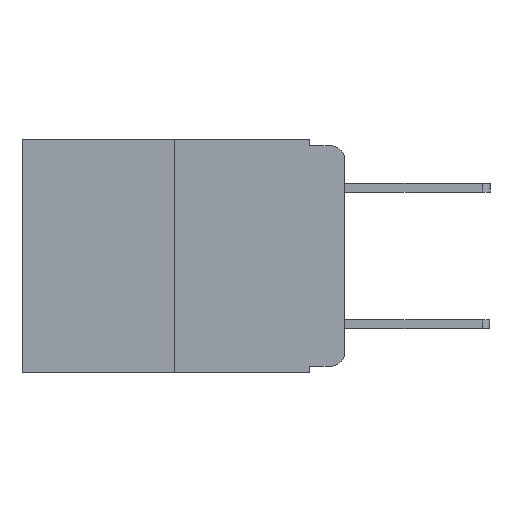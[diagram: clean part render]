
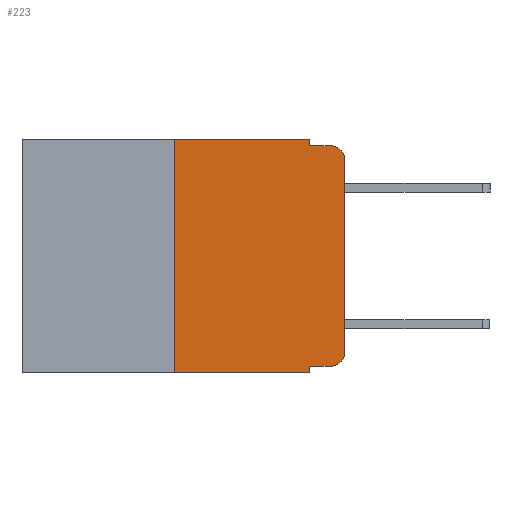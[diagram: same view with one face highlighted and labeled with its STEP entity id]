
A CAD part, left-side view. The second image highlights one B-rep face of the part: STEP entity #223.
In plain terms, the highlighted planar face has unit normal (-1, 0, 0).
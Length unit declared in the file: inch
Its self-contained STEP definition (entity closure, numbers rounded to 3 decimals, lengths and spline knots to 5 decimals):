
#196 = CARTESIAN_POINT ( 'NONE',  ( 0., 0.473, -0.343 ) ) ;
#216 = VERTEX_POINT ( 'NONE', #3638 ) ;
#223 = ADVANCED_FACE ( 'NONE', ( #1597 ), #9440, .F. ) ;
#251 = VERTEX_POINT ( 'NONE', #6476 ) ;
#408 = CARTESIAN_POINT ( 'NONE',  ( 0., 0.051, -0.01 ) ) ;
#806 = EDGE_CURVE ( 'NONE', #216, #2228, #10338, .T. ) ;
#811 = ORIENTED_EDGE ( 'NONE', *, *, #6741, .F. ) ;
#897 = DIRECTION ( 'NONE',  ( -1., 0., 0. ) ) ;
#949 = AXIS2_PLACEMENT_3D ( 'NONE', #9639, #4742, #10482 ) ;
#1180 = EDGE_CURVE ( 'NONE', #251, #8463, #7514, .T. ) ;
#1597 = FACE_OUTER_BOUND ( 'NONE', #4445, .T. ) ;
#1632 = LINE ( 'NONE', #1672, #9632 ) ;
#1672 = CARTESIAN_POINT ( 'NONE',  ( 0., 0.051, -0.01 ) ) ;
#1817 = CARTESIAN_POINT ( 'NONE',  ( 0., 0.02, -0.313 ) ) ;
#1845 = AXIS2_PLACEMENT_3D ( 'NONE', #7605, #2229, #7422 ) ;
#1893 = CARTESIAN_POINT ( 'NONE',  ( 0., 0.051, 0. ) ) ;
#1928 = CARTESIAN_POINT ( 'NONE',  ( 0., 0.051, -0.333 ) ) ;
#2087 = ORIENTED_EDGE ( 'NONE', *, *, #3782, .T. ) ;
#2106 = VECTOR ( 'NONE', #9404, 39.37008 ) ;
#2228 = VERTEX_POINT ( 'NONE', #7787 ) ;
#2229 = DIRECTION ( 'NONE',  ( 1., 0., 0. ) ) ;
#2386 = ORIENTED_EDGE ( 'NONE', *, *, #806, .F. ) ;
#2463 = DIRECTION ( 'NONE',  ( 0., -1., 0. ) ) ;
#2829 = DIRECTION ( 'NONE',  ( 0., 0., -1. ) ) ;
#2911 = VECTOR ( 'NONE', #5939, 39.37008 ) ;
#3011 = CARTESIAN_POINT ( 'NONE',  ( 0., 0., -0.313 ) ) ;
#3073 = VECTOR ( 'NONE', #9023, 39.37008 ) ;
#3480 = DIRECTION ( 'NONE',  ( 0., -1., 0. ) ) ;
#3638 = CARTESIAN_POINT ( 'NONE',  ( 0., 0.25, 0. ) ) ;
#3747 = VERTEX_POINT ( 'NONE', #6736 ) ;
#3782 = EDGE_CURVE ( 'NONE', #6854, #10087, #6702, .T. ) ;
#3838 = CIRCLE ( 'NONE', #949, 0.02 ) ;
#3851 = VECTOR ( 'NONE', #3480, 39.37008 ) ;
#4028 = CARTESIAN_POINT ( 'NONE',  ( 0., 0.051, 0. ) ) ;
#4170 = EDGE_CURVE ( 'NONE', #5185, #3747, #1632, .T. ) ;
#4412 = AXIS2_PLACEMENT_3D ( 'NONE', #1817, #897, #10170 ) ;
#4445 = EDGE_LOOP ( 'NONE', ( #8730, #10282, #5439, #811, #2386, #7401, #9883, #6822, #10832, #2087 ) ) ;
#4742 = DIRECTION ( 'NONE',  ( -1., 0., 0. ) ) ;
#4751 = EDGE_CURVE ( 'NONE', #4864, #216, #5285, .T. ) ;
#4757 = CARTESIAN_POINT ( 'NONE',  ( 0., 0.02, -0.333 ) ) ;
#4864 = VERTEX_POINT ( 'NONE', #6947 ) ;
#5097 = VECTOR ( 'NONE', #2829, 39.37008 ) ;
#5185 = VERTEX_POINT ( 'NONE', #408 ) ;
#5285 = LINE ( 'NONE', #7669, #2911 ) ;
#5436 = LINE ( 'NONE', #8190, #3073 ) ;
#5439 = ORIENTED_EDGE ( 'NONE', *, *, #4170, .F. ) ;
#5939 = DIRECTION ( 'NONE',  ( 0., 0., 1. ) ) ;
#6011 = VECTOR ( 'NONE', #2463, 39.37008 ) ;
#6476 = CARTESIAN_POINT ( 'NONE',  ( 0., 0.051, -0.333 ) ) ;
#6702 = CIRCLE ( 'NONE', #4412, 0.02 ) ;
#6736 = CARTESIAN_POINT ( 'NONE',  ( 0., 0.02, -0.01 ) ) ;
#6741 = EDGE_CURVE ( 'NONE', #2228, #5185, #10964, .T. ) ;
#6822 = ORIENTED_EDGE ( 'NONE', *, *, #1180, .F. ) ;
#6854 = VERTEX_POINT ( 'NONE', #4757 ) ;
#6899 = VECTOR ( 'NONE', #8946, 39.37008 ) ;
#6947 = CARTESIAN_POINT ( 'NONE',  ( 0., 0.25, -0.343 ) ) ;
#7375 = EDGE_CURVE ( 'NONE', #251, #6854, #9168, .T. ) ;
#7401 = ORIENTED_EDGE ( 'NONE', *, *, #4751, .F. ) ;
#7422 = DIRECTION ( 'NONE',  ( 0., 0., -1. ) ) ;
#7474 = EDGE_CURVE ( 'NONE', #4864, #8463, #8238, .T. ) ;
#7514 = LINE ( 'NONE', #4028, #5097 ) ;
#7605 = CARTESIAN_POINT ( 'NONE',  ( 0., 0.473, 0. ) ) ;
#7669 = CARTESIAN_POINT ( 'NONE',  ( 0., 0.25, 0. ) ) ;
#7787 = CARTESIAN_POINT ( 'NONE',  ( 0., 0.051, 0. ) ) ;
#7907 = EDGE_CURVE ( 'NONE', #9501, #3747, #3838, .T. ) ;
#7925 = CARTESIAN_POINT ( 'NONE',  ( 0., 0., -0.03 ) ) ;
#8190 = CARTESIAN_POINT ( 'NONE',  ( 0., 0., 0. ) ) ;
#8238 = LINE ( 'NONE', #196, #3851 ) ;
#8317 = CARTESIAN_POINT ( 'NONE',  ( 0., 0.051, -0.343 ) ) ;
#8463 = VERTEX_POINT ( 'NONE', #8317 ) ;
#8730 = ORIENTED_EDGE ( 'NONE', *, *, #9913, .T. ) ;
#8946 = DIRECTION ( 'NONE',  ( 0., 0., -1. ) ) ;
#9023 = DIRECTION ( 'NONE',  ( 0., 0., 1. ) ) ;
#9168 = LINE ( 'NONE', #1928, #2106 ) ;
#9404 = DIRECTION ( 'NONE',  ( 0., -1., 0. ) ) ;
#9440 = PLANE ( 'NONE',  #1845 ) ;
#9501 = VERTEX_POINT ( 'NONE', #7925 ) ;
#9632 = VECTOR ( 'NONE', #10300, 39.37008 ) ;
#9639 = CARTESIAN_POINT ( 'NONE',  ( 0., 0.02, -0.03 ) ) ;
#9883 = ORIENTED_EDGE ( 'NONE', *, *, #7474, .T. ) ;
#9913 = EDGE_CURVE ( 'NONE', #10087, #9501, #5436, .T. ) ;
#10087 = VERTEX_POINT ( 'NONE', #3011 ) ;
#10163 = CARTESIAN_POINT ( 'NONE',  ( 0., 0.473, 0. ) ) ;
#10170 = DIRECTION ( 'NONE',  ( 0., 0., -1. ) ) ;
#10282 = ORIENTED_EDGE ( 'NONE', *, *, #7907, .T. ) ;
#10300 = DIRECTION ( 'NONE',  ( 0., -1., 0. ) ) ;
#10338 = LINE ( 'NONE', #10163, #6011 ) ;
#10482 = DIRECTION ( 'NONE',  ( 0., 0., -1. ) ) ;
#10832 = ORIENTED_EDGE ( 'NONE', *, *, #7375, .T. ) ;
#10964 = LINE ( 'NONE', #1893, #6899 ) ;
